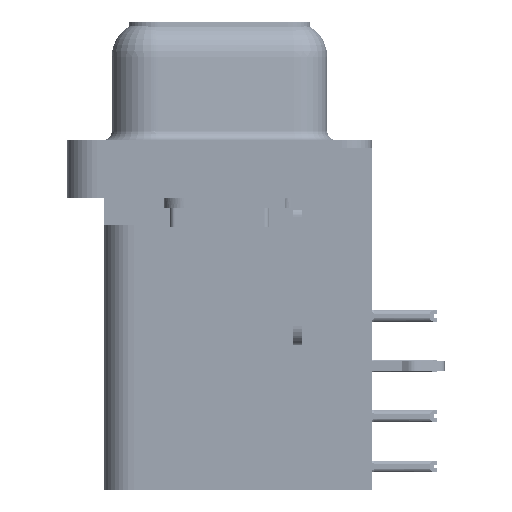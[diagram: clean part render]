
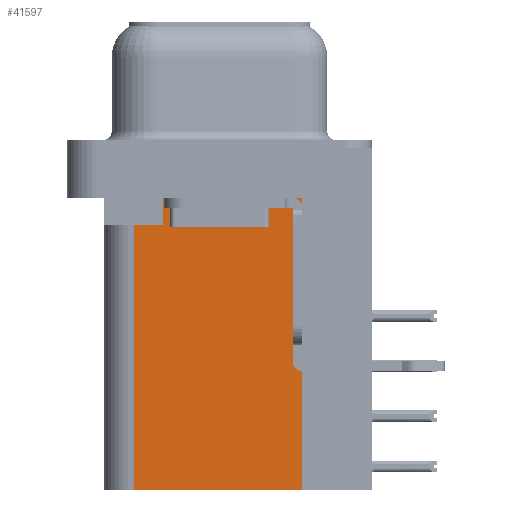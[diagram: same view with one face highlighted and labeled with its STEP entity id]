
A CAD part, left-side view. The second image highlights one B-rep face of the part: STEP entity #41597.
In plain terms, the highlighted planar face has unit normal (-1, 0, 0).
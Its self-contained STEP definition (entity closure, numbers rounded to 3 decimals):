
#2015 = VERTEX_POINT ( 'NONE', #15100 ) ;
#4700 = VECTOR ( 'NONE', #21892, 1000. ) ;
#5052 = CARTESIAN_POINT ( 'NONE',  ( 3.75, -4.2, -17.3 ) ) ;
#6295 = VECTOR ( 'NONE', #27715, 1000. ) ;
#6506 = EDGE_CURVE ( 'NONE', #2015, #45285, #13633, .T. ) ;
#7634 = DIRECTION ( 'NONE',  ( 1., 0., 0. ) ) ;
#7918 = DIRECTION ( 'NONE',  ( 0., 0., -1. ) ) ;
#8543 = DIRECTION ( 'NONE',  ( 0., 1., 0. ) ) ;
#9146 = ORIENTED_EDGE ( 'NONE', *, *, #37963, .T. ) ;
#10397 = FACE_OUTER_BOUND ( 'NONE', #40944, .T. ) ;
#13436 = CARTESIAN_POINT ( 'NONE',  ( 3.75, 2.85, -3.9 ) ) ;
#13633 = LINE ( 'NONE', #19520, #35900 ) ;
#13891 = ORIENTED_EDGE ( 'NONE', *, *, #6506, .T. ) ;
#13945 = DIRECTION ( 'NONE',  ( 0., 1., 0. ) ) ;
#15100 = CARTESIAN_POINT ( 'NONE',  ( 3.75, -4.2, -2.5 ) ) ;
#19520 = CARTESIAN_POINT ( 'NONE',  ( 3.75, -4.2, -2.5 ) ) ;
#20817 = VERTEX_POINT ( 'NONE', #68143 ) ;
#21123 = EDGE_CURVE ( 'NONE', #20817, #45914, #33849, .T. ) ;
#21892 = DIRECTION ( 'NONE',  ( 0., 1., 0. ) ) ;
#24800 = EDGE_CURVE ( 'NONE', #20817, #2015, #45490, .T. ) ;
#24830 = ORIENTED_EDGE ( 'NONE', *, *, #69291, .F. ) ;
#27715 = DIRECTION ( 'NONE',  ( 0., 0., 1. ) ) ;
#27763 = EDGE_CURVE ( 'NONE', #45285, #55686, #63972, .T. ) ;
#28574 = CARTESIAN_POINT ( 'NONE',  ( 3.75, 4.35, -17.3 ) ) ;
#30363 = CARTESIAN_POINT ( 'NONE',  ( 3.75, 2.85, -3.9 ) ) ;
#30387 = ORIENTED_EDGE ( 'NONE', *, *, #21123, .F. ) ;
#33050 = VECTOR ( 'NONE', #7918, 1000. ) ;
#33609 = VERTEX_POINT ( 'NONE', #35031 ) ;
#33849 = LINE ( 'NONE', #60204, #4700 ) ;
#35031 = CARTESIAN_POINT ( 'NONE',  ( 3.75, 4.35, -3.9 ) ) ;
#35900 = VECTOR ( 'NONE', #13945, 1000. ) ;
#37963 = EDGE_CURVE ( 'NONE', #55686, #33609, #51059, .T. ) ;
#38622 = DIRECTION ( 'NONE',  ( 0., 0., 1. ) ) ;
#40492 = PLANE ( 'NONE',  #44172 ) ;
#40944 = EDGE_LOOP ( 'NONE', ( #13891, #67528, #9146, #24830, #30387, #47915 ) ) ;
#41597 = ADVANCED_FACE ( 'NONE', ( #10397 ), #40492, .F. ) ;
#42027 = VECTOR ( 'NONE', #38622, 1000. ) ;
#44172 = AXIS2_PLACEMENT_3D ( 'NONE', #67836, #7634, #46046 ) ;
#45285 = VERTEX_POINT ( 'NONE', #45466 ) ;
#45466 = CARTESIAN_POINT ( 'NONE',  ( 3.75, 2.85, -2.5 ) ) ;
#45490 = LINE ( 'NONE', #5052, #42027 ) ;
#45914 = VERTEX_POINT ( 'NONE', #28574 ) ;
#46046 = DIRECTION ( 'NONE',  ( 0., 1., 0. ) ) ;
#47915 = ORIENTED_EDGE ( 'NONE', *, *, #24800, .T. ) ;
#49350 = VECTOR ( 'NONE', #8543, 1000. ) ;
#51059 = LINE ( 'NONE', #52444, #49350 ) ;
#51843 = LINE ( 'NONE', #55040, #6295 ) ;
#52444 = CARTESIAN_POINT ( 'NONE',  ( 3.75, 0., -3.9 ) ) ;
#55040 = CARTESIAN_POINT ( 'NONE',  ( 3.75, 4.35, -17.3 ) ) ;
#55686 = VERTEX_POINT ( 'NONE', #30363 ) ;
#60204 = CARTESIAN_POINT ( 'NONE',  ( 3.75, -4.2, -17.3 ) ) ;
#63972 = LINE ( 'NONE', #13436, #33050 ) ;
#67528 = ORIENTED_EDGE ( 'NONE', *, *, #27763, .T. ) ;
#67836 = CARTESIAN_POINT ( 'NONE',  ( 3.75, -4.2, -17.3 ) ) ;
#68143 = CARTESIAN_POINT ( 'NONE',  ( 3.75, -4.2, -17.3 ) ) ;
#69291 = EDGE_CURVE ( 'NONE', #45914, #33609, #51843, .T. ) ;
